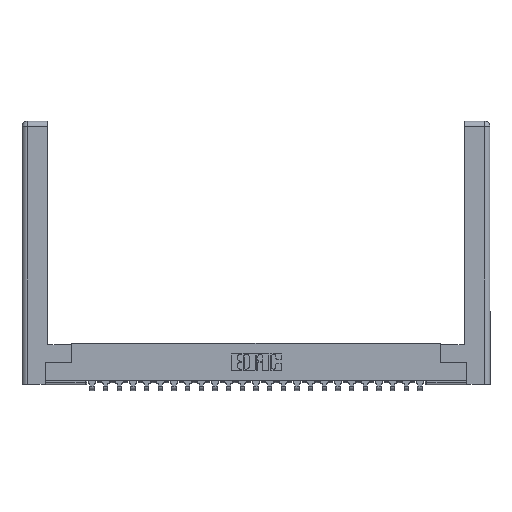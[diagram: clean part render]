
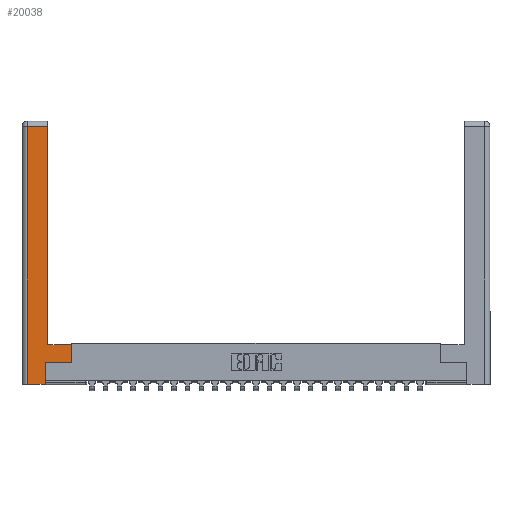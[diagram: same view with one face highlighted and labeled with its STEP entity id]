
A CAD part, top view. The second image highlights one B-rep face of the part: STEP entity #20038.
In plain terms, the highlighted planar face has unit normal (0, 0, 1).
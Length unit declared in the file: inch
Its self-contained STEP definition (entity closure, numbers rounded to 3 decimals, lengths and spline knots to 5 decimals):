
#335 = DIRECTION ( 'NONE',  ( 0., 1., 0. ) ) ;
#841 = VERTEX_POINT ( 'NONE', #18957 ) ;
#1119 = VECTOR ( 'NONE', #17246, 39.37008 ) ;
#1352 = CARTESIAN_POINT ( 'NONE',  ( 0.295, 0.45, 0. ) ) ;
#1479 = LINE ( 'NONE', #1352, #7867 ) ;
#1688 = LINE ( 'NONE', #24386, #7365 ) ;
#2034 = VERTEX_POINT ( 'NONE', #4248 ) ;
#2803 = CARTESIAN_POINT ( 'NONE',  ( 0.565, 0.245, 0. ) ) ;
#3185 = DIRECTION ( 'NONE',  ( 0., -1., 0. ) ) ;
#3285 = CARTESIAN_POINT ( 'NONE',  ( 0.565, 0.45, 0. ) ) ;
#3628 = LINE ( 'NONE', #19710, #8115 ) ;
#4248 = CARTESIAN_POINT ( 'NONE',  ( 0.265, 0.245, 0. ) ) ;
#5477 = PLANE ( 'NONE',  #11230 ) ;
#6076 = CARTESIAN_POINT ( 'NONE',  ( 0.0615, 2.94, 0. ) ) ;
#7318 = ORIENTED_EDGE ( 'NONE', *, *, #11932, .T. ) ;
#7365 = VECTOR ( 'NONE', #16015, 39.37008 ) ;
#7867 = VECTOR ( 'NONE', #20059, 39.37008 ) ;
#7950 = LINE ( 'NONE', #22558, #23966 ) ;
#8091 = DIRECTION ( 'NONE',  ( 1., 0., 0. ) ) ;
#8115 = VECTOR ( 'NONE', #25701, 39.37008 ) ;
#8188 = CARTESIAN_POINT ( 'NONE',  ( 0.265, 0.245, 0. ) ) ;
#8248 = EDGE_CURVE ( 'NONE', #24045, #15567, #3628, .T. ) ;
#9085 = VECTOR ( 'NONE', #11274, 39.37008 ) ;
#9556 = LINE ( 'NONE', #3285, #9085 ) ;
#9882 = CARTESIAN_POINT ( 'NONE',  ( 0., 0., 0. ) ) ;
#9919 = CARTESIAN_POINT ( 'NONE',  ( 0.0615, 0., 0. ) ) ;
#10003 = DIRECTION ( 'NONE',  ( 0., 0., -1. ) ) ;
#10687 = CARTESIAN_POINT ( 'NONE',  ( 0.265, 0., 0. ) ) ;
#10939 = VECTOR ( 'NONE', #3185, 39.37008 ) ;
#11170 = CARTESIAN_POINT ( 'NONE',  ( 0.0615, 0., 0. ) ) ;
#11230 = AXIS2_PLACEMENT_3D ( 'NONE', #9882, #10003, #15957 ) ;
#11274 = DIRECTION ( 'NONE',  ( 0., 1., 0. ) ) ;
#11407 = ORIENTED_EDGE ( 'NONE', *, *, #12010, .T. ) ;
#11932 = EDGE_CURVE ( 'NONE', #18980, #24081, #9556, .T. ) ;
#12004 = ORIENTED_EDGE ( 'NONE', *, *, #21658, .T. ) ;
#12010 = EDGE_CURVE ( 'NONE', #2034, #18980, #1688, .T. ) ;
#13540 = LINE ( 'NONE', #11170, #10939 ) ;
#15007 = ORIENTED_EDGE ( 'NONE', *, *, #8248, .T. ) ;
#15431 = EDGE_CURVE ( 'NONE', #15567, #26257, #13540, .T. ) ;
#15544 = CARTESIAN_POINT ( 'NONE',  ( 0.295, 2.94, 0. ) ) ;
#15567 = VERTEX_POINT ( 'NONE', #6076 ) ;
#15779 = EDGE_LOOP ( 'NONE', ( #16340, #15007, #21920, #24323, #18942, #11407, #7318, #12004 ) ) ;
#15957 = DIRECTION ( 'NONE',  ( -1., 0., 0. ) ) ;
#16015 = DIRECTION ( 'NONE',  ( 1., 0., 0. ) ) ;
#16340 = ORIENTED_EDGE ( 'NONE', *, *, #21934, .T. ) ;
#17246 = DIRECTION ( 'NONE',  ( 0., 1., 0. ) ) ;
#17829 = FACE_OUTER_BOUND ( 'NONE', #15779, .T. ) ;
#18546 = LINE ( 'NONE', #8188, #26277 ) ;
#18942 = ORIENTED_EDGE ( 'NONE', *, *, #24597, .T. ) ;
#18957 = CARTESIAN_POINT ( 'NONE',  ( 0.295, 0.45, 0. ) ) ;
#18980 = VERTEX_POINT ( 'NONE', #2803 ) ;
#19371 = LINE ( 'NONE', #24963, #1119 ) ;
#19710 = CARTESIAN_POINT ( 'NONE',  ( 0.0615, 2.94, 0. ) ) ;
#20038 = ADVANCED_FACE ( 'NONE', ( #17829 ), #5477, .F. ) ;
#20059 = DIRECTION ( 'NONE',  ( -1., 0., 0. ) ) ;
#20575 = EDGE_CURVE ( 'NONE', #26257, #23383, #7950, .T. ) ;
#21658 = EDGE_CURVE ( 'NONE', #24081, #841, #1479, .T. ) ;
#21920 = ORIENTED_EDGE ( 'NONE', *, *, #15431, .T. ) ;
#21934 = EDGE_CURVE ( 'NONE', #841, #24045, #19371, .T. ) ;
#22558 = CARTESIAN_POINT ( 'NONE',  ( 0.265, 0., 0. ) ) ;
#23383 = VERTEX_POINT ( 'NONE', #10687 ) ;
#23966 = VECTOR ( 'NONE', #8091, 39.37008 ) ;
#24045 = VERTEX_POINT ( 'NONE', #15544 ) ;
#24081 = VERTEX_POINT ( 'NONE', #24554 ) ;
#24323 = ORIENTED_EDGE ( 'NONE', *, *, #20575, .T. ) ;
#24386 = CARTESIAN_POINT ( 'NONE',  ( 0.565, 0.245, 0. ) ) ;
#24554 = CARTESIAN_POINT ( 'NONE',  ( 0.565, 0.45, 0. ) ) ;
#24597 = EDGE_CURVE ( 'NONE', #23383, #2034, #18546, .T. ) ;
#24963 = CARTESIAN_POINT ( 'NONE',  ( 0.295, 3., 0. ) ) ;
#25701 = DIRECTION ( 'NONE',  ( -1., 0., 0. ) ) ;
#26257 = VERTEX_POINT ( 'NONE', #9919 ) ;
#26277 = VECTOR ( 'NONE', #335, 39.37008 ) ;
